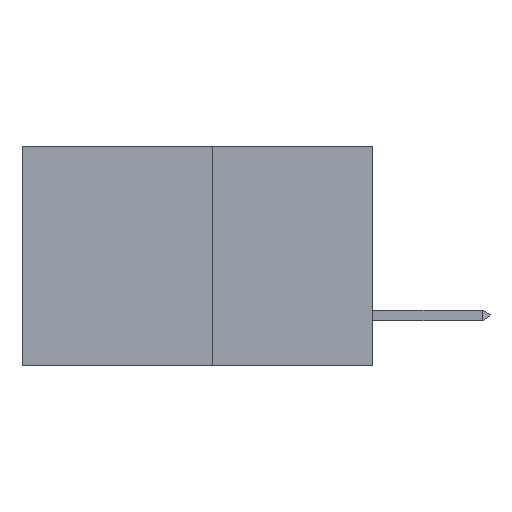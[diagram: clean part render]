
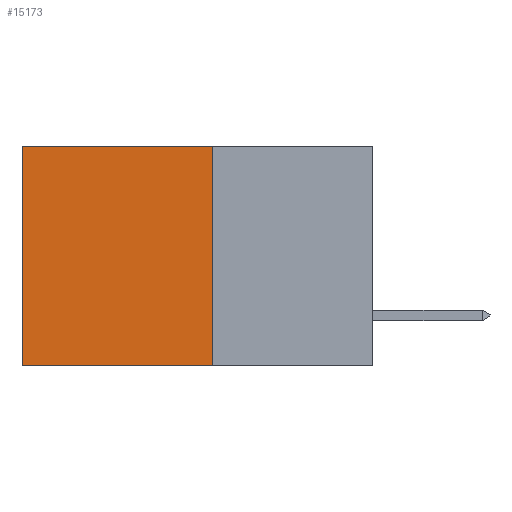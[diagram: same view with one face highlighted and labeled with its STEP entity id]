
A CAD part, left-side view. The second image highlights one B-rep face of the part: STEP entity #15173.
In plain terms, the highlighted planar face has unit normal (-1, 0, 0).
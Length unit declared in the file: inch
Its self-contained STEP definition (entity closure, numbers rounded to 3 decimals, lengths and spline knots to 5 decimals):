
#282 = VERTEX_POINT ( 'NONE', #14077 ) ;
#778 = LINE ( 'NONE', #1686, #7628 ) ;
#1205 = VERTEX_POINT ( 'NONE', #12511 ) ;
#1686 = CARTESIAN_POINT ( 'NONE',  ( 0.277, 0.27, -0.37 ) ) ;
#1774 = CARTESIAN_POINT ( 'NONE',  ( 0.277, 0.59, -0.37 ) ) ;
#1893 = ORIENTED_EDGE ( 'NONE', *, *, #3498, .T. ) ;
#2050 = VERTEX_POINT ( 'NONE', #9213 ) ;
#2492 = CARTESIAN_POINT ( 'NONE',  ( 0.277, 0.27, 0. ) ) ;
#3176 = DIRECTION ( 'NONE',  ( 0., 1., 0. ) ) ;
#3187 = DIRECTION ( 'NONE',  ( 0., 0., -1. ) ) ;
#3498 = EDGE_CURVE ( 'NONE', #9688, #1205, #7886, .T. ) ;
#4841 = EDGE_CURVE ( 'NONE', #1205, #282, #10028, .T. ) ;
#5690 = PLANE ( 'NONE',  #6516 ) ;
#5811 = CARTESIAN_POINT ( 'NONE',  ( 0.277, 0.27, -0.37 ) ) ;
#6516 = AXIS2_PLACEMENT_3D ( 'NONE', #5811, #15529, #8340 ) ;
#7160 = VECTOR ( 'NONE', #3176, 39.37008 ) ;
#7628 = VECTOR ( 'NONE', #12055, 39.37008 ) ;
#7886 = LINE ( 'NONE', #2492, #7160 ) ;
#8340 = DIRECTION ( 'NONE',  ( 0., 0., -1. ) ) ;
#8854 = EDGE_CURVE ( 'NONE', #9688, #2050, #778, .T. ) ;
#9213 = CARTESIAN_POINT ( 'NONE',  ( 0.277, 0.27, -0.37 ) ) ;
#9688 = VERTEX_POINT ( 'NONE', #11923 ) ;
#10028 = LINE ( 'NONE', #1774, #16020 ) ;
#10039 = LINE ( 'NONE', #16486, #13824 ) ;
#10541 = DIRECTION ( 'NONE',  ( 0., 1., 0. ) ) ;
#11069 = ORIENTED_EDGE ( 'NONE', *, *, #8854, .F. ) ;
#11188 = ORIENTED_EDGE ( 'NONE', *, *, #4841, .T. ) ;
#11520 = EDGE_CURVE ( 'NONE', #2050, #282, #10039, .T. ) ;
#11923 = CARTESIAN_POINT ( 'NONE',  ( 0.277, 0.27, 0. ) ) ;
#12055 = DIRECTION ( 'NONE',  ( 0., 0., -1. ) ) ;
#12200 = ORIENTED_EDGE ( 'NONE', *, *, #11520, .F. ) ;
#12511 = CARTESIAN_POINT ( 'NONE',  ( 0.277, 0.59, 0. ) ) ;
#13824 = VECTOR ( 'NONE', #10541, 39.37008 ) ;
#14077 = CARTESIAN_POINT ( 'NONE',  ( 0.277, 0.59, -0.37 ) ) ;
#14187 = EDGE_LOOP ( 'NONE', ( #11188, #12200, #11069, #1893 ) ) ;
#15173 = ADVANCED_FACE ( 'NONE', ( #16511 ), #5690, .F. ) ;
#15529 = DIRECTION ( 'NONE',  ( 1., 0., 0. ) ) ;
#16020 = VECTOR ( 'NONE', #3187, 39.37008 ) ;
#16486 = CARTESIAN_POINT ( 'NONE',  ( 0.277, 0.27, -0.37 ) ) ;
#16511 = FACE_OUTER_BOUND ( 'NONE', #14187, .T. ) ;
